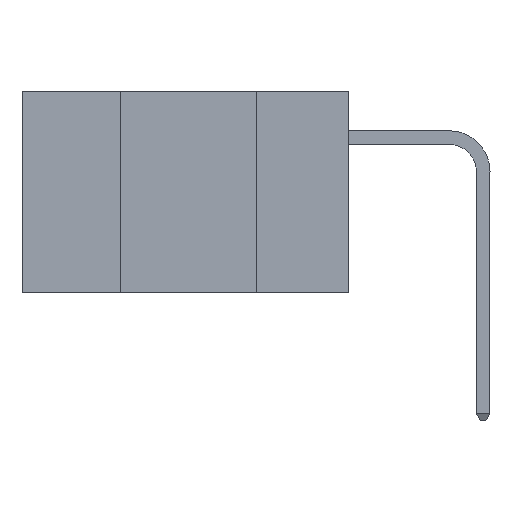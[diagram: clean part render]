
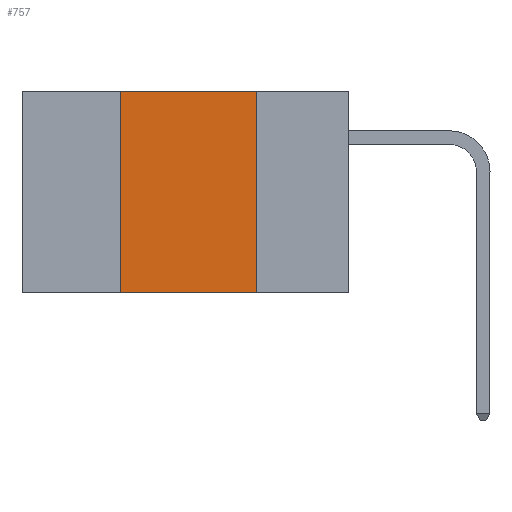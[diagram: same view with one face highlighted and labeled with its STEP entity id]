
A CAD part, left-side view. The second image highlights one B-rep face of the part: STEP entity #757.
In plain terms, the highlighted planar face has unit normal (-1, 0, 0).
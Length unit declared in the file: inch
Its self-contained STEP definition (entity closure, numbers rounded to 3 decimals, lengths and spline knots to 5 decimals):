
#43 = EDGE_CURVE ( 'NONE', #20985, #13318, #13142, .T. ) ;
#393 = CARTESIAN_POINT ( 'NONE',  ( 0., 0.17, 0. ) ) ;
#757 = ADVANCED_FACE ( 'NONE', ( #6171 ), #23545, .F. ) ;
#1545 = VERTEX_POINT ( 'NONE', #9385 ) ;
#1600 = CARTESIAN_POINT ( 'NONE',  ( 0., 0.42, 0. ) ) ;
#2118 = DIRECTION ( 'NONE',  ( 0., -1., 0. ) ) ;
#2717 = CARTESIAN_POINT ( 'NONE',  ( 0., 0.17, -0.37 ) ) ;
#2879 = VECTOR ( 'NONE', #3630, 39.37008 ) ;
#3630 = DIRECTION ( 'NONE',  ( 0., 0., 1. ) ) ;
#5026 = VECTOR ( 'NONE', #6091, 39.37008 ) ;
#5891 = VECTOR ( 'NONE', #2118, 39.37008 ) ;
#6091 = DIRECTION ( 'NONE',  ( 0., 0., -1. ) ) ;
#6171 = FACE_OUTER_BOUND ( 'NONE', #23228, .T. ) ;
#6307 = LINE ( 'NONE', #21840, #5026 ) ;
#7811 = VECTOR ( 'NONE', #16810, 39.37008 ) ;
#8330 = LINE ( 'NONE', #1600, #2879 ) ;
#9385 = CARTESIAN_POINT ( 'NONE',  ( 0., 0.42, 0. ) ) ;
#9662 = ORIENTED_EDGE ( 'NONE', *, *, #12428, .F. ) ;
#12142 = CARTESIAN_POINT ( 'NONE',  ( 0., 0.6, 0. ) ) ;
#12428 = EDGE_CURVE ( 'NONE', #20985, #1545, #8330, .T. ) ;
#13142 = LINE ( 'NONE', #15049, #7811 ) ;
#13318 = VERTEX_POINT ( 'NONE', #2717 ) ;
#13754 = ORIENTED_EDGE ( 'NONE', *, *, #16317, .F. ) ;
#13763 = EDGE_CURVE ( 'NONE', #19972, #13318, #6307, .T. ) ;
#15049 = CARTESIAN_POINT ( 'NONE',  ( 0., 0.6, -0.37 ) ) ;
#16317 = EDGE_CURVE ( 'NONE', #1545, #19972, #17079, .T. ) ;
#16410 = AXIS2_PLACEMENT_3D ( 'NONE', #23164, #23648, #23864 ) ;
#16810 = DIRECTION ( 'NONE',  ( 0., -1., 0. ) ) ;
#17079 = LINE ( 'NONE', #12142, #5891 ) ;
#19972 = VERTEX_POINT ( 'NONE', #393 ) ;
#20985 = VERTEX_POINT ( 'NONE', #23000 ) ;
#21840 = CARTESIAN_POINT ( 'NONE',  ( 0., 0.17, 0. ) ) ;
#23000 = CARTESIAN_POINT ( 'NONE',  ( 0., 0.42, -0.37 ) ) ;
#23164 = CARTESIAN_POINT ( 'NONE',  ( 0., 0.6, 0. ) ) ;
#23228 = EDGE_LOOP ( 'NONE', ( #23777, #13754, #9662, #24839 ) ) ;
#23545 = PLANE ( 'NONE',  #16410 ) ;
#23648 = DIRECTION ( 'NONE',  ( 1., 0., 0. ) ) ;
#23777 = ORIENTED_EDGE ( 'NONE', *, *, #13763, .F. ) ;
#23864 = DIRECTION ( 'NONE',  ( 0., 0., -1. ) ) ;
#24839 = ORIENTED_EDGE ( 'NONE', *, *, #43, .T. ) ;
